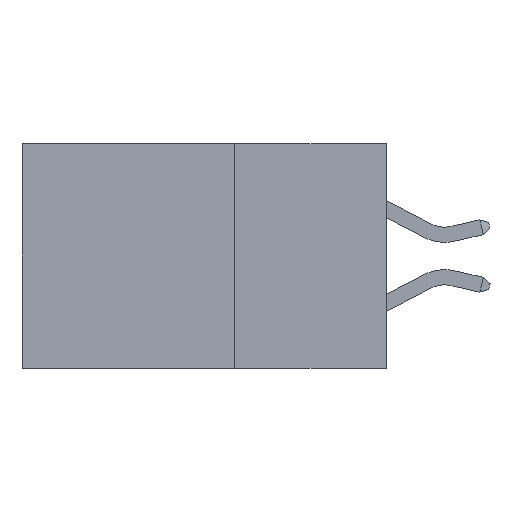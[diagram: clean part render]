
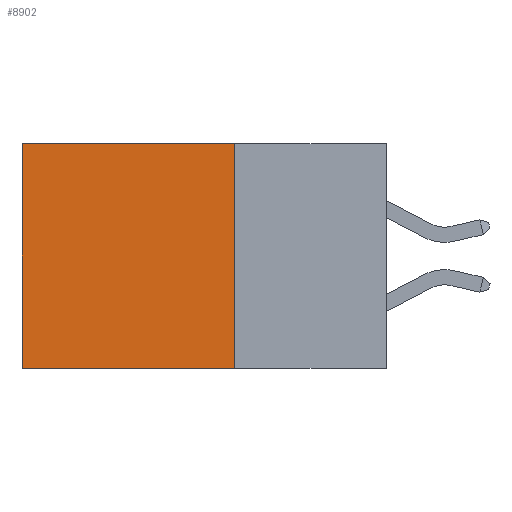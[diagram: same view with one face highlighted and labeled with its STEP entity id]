
A CAD part, left-side view. The second image highlights one B-rep face of the part: STEP entity #8902.
In plain terms, the highlighted planar face has unit normal (-1, 0, 0).
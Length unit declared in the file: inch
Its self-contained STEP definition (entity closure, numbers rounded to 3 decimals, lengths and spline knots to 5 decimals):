
#118 = AXIS2_PLACEMENT_3D ( 'NONE', #14207, #2458, #5101 ) ;
#668 = EDGE_CURVE ( 'NONE', #10061, #8009, #3568, .T. ) ;
#1796 = CARTESIAN_POINT ( 'NONE',  ( 0.298, 0.6, -0.37 ) ) ;
#2458 = DIRECTION ( 'NONE',  ( 1., 0., 0. ) ) ;
#2655 = FACE_OUTER_BOUND ( 'NONE', #10687, .T. ) ;
#3071 = CARTESIAN_POINT ( 'NONE',  ( 0.298, 0.25, 0. ) ) ;
#3194 = EDGE_CURVE ( 'NONE', #10061, #14268, #5488, .T. ) ;
#3568 = LINE ( 'NONE', #7233, #4384 ) ;
#4384 = VECTOR ( 'NONE', #6102, 39.37008 ) ;
#5101 = DIRECTION ( 'NONE',  ( 0., 0., -1. ) ) ;
#5488 = LINE ( 'NONE', #3071, #13337 ) ;
#5677 = DIRECTION ( 'NONE',  ( 0., 1., 0. ) ) ;
#6009 = VERTEX_POINT ( 'NONE', #1796 ) ;
#6102 = DIRECTION ( 'NONE',  ( 0., 1., 0. ) ) ;
#6439 = LINE ( 'NONE', #7778, #15705 ) ;
#6523 = CARTESIAN_POINT ( 'NONE',  ( 0.298, 0.25, -0.37 ) ) ;
#6996 = ORIENTED_EDGE ( 'NONE', *, *, #7994, .T. ) ;
#7233 = CARTESIAN_POINT ( 'NONE',  ( 0.298, 0.25, 0. ) ) ;
#7578 = PLANE ( 'NONE',  #118 ) ;
#7778 = CARTESIAN_POINT ( 'NONE',  ( 0.298, 0.6, 0. ) ) ;
#7994 = EDGE_CURVE ( 'NONE', #8009, #6009, #6439, .T. ) ;
#8009 = VERTEX_POINT ( 'NONE', #15706 ) ;
#8902 = ADVANCED_FACE ( 'NONE', ( #2655 ), #7578, .F. ) ;
#9212 = DIRECTION ( 'NONE',  ( 0., 0., -1. ) ) ;
#9542 = CARTESIAN_POINT ( 'NONE',  ( 0.298, 0.25, -0.37 ) ) ;
#10061 = VERTEX_POINT ( 'NONE', #14175 ) ;
#10687 = EDGE_LOOP ( 'NONE', ( #6996, #16521, #13358, #15527 ) ) ;
#11839 = VECTOR ( 'NONE', #5677, 39.37008 ) ;
#12209 = LINE ( 'NONE', #9542, #11839 ) ;
#13337 = VECTOR ( 'NONE', #14729, 39.37008 ) ;
#13358 = ORIENTED_EDGE ( 'NONE', *, *, #3194, .F. ) ;
#14175 = CARTESIAN_POINT ( 'NONE',  ( 0.298, 0.25, 0. ) ) ;
#14207 = CARTESIAN_POINT ( 'NONE',  ( 0.298, 0.25, 0. ) ) ;
#14268 = VERTEX_POINT ( 'NONE', #6523 ) ;
#14729 = DIRECTION ( 'NONE',  ( 0., 0., -1. ) ) ;
#15527 = ORIENTED_EDGE ( 'NONE', *, *, #668, .T. ) ;
#15705 = VECTOR ( 'NONE', #9212, 39.37008 ) ;
#15706 = CARTESIAN_POINT ( 'NONE',  ( 0.298, 0.6, 0. ) ) ;
#16186 = EDGE_CURVE ( 'NONE', #14268, #6009, #12209, .T. ) ;
#16521 = ORIENTED_EDGE ( 'NONE', *, *, #16186, .F. ) ;
